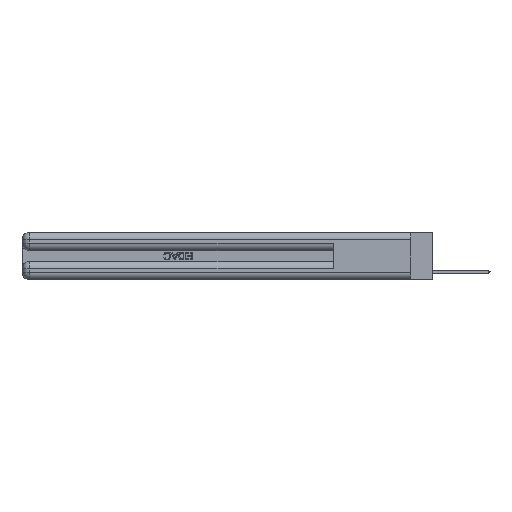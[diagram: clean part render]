
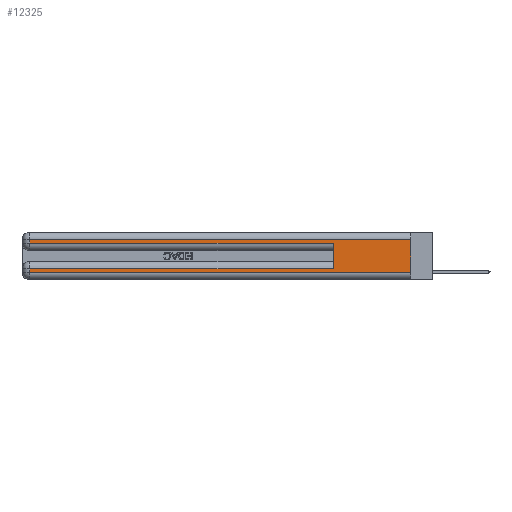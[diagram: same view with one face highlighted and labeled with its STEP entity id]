
A CAD part, left-side view. The second image highlights one B-rep face of the part: STEP entity #12325.
In plain terms, the highlighted planar face has unit normal (-1, 0, 0).
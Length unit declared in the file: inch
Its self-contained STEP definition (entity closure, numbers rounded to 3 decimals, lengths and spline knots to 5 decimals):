
#663 = VERTEX_POINT ( 'NONE', #5618 ) ;
#2014 = VERTEX_POINT ( 'NONE', #27838 ) ;
#2231 = ORIENTED_EDGE ( 'NONE', *, *, #29048, .F. ) ;
#2716 = EDGE_CURVE ( 'NONE', #2014, #30190, #10876, .T. ) ;
#3469 = LINE ( 'NONE', #19719, #8461 ) ;
#3777 = LINE ( 'NONE', #14670, #31603 ) ;
#3831 = DIRECTION ( 'NONE',  ( 0., -1., 0. ) ) ;
#4445 = DIRECTION ( 'NONE',  ( 0., 1., 0. ) ) ;
#5618 = CARTESIAN_POINT ( 'NONE',  ( 0., 0., 0.31 ) ) ;
#5751 = EDGE_CURVE ( 'NONE', #25870, #30190, #3469, .T. ) ;
#5931 = CARTESIAN_POINT ( 'NONE',  ( 0., 0.6, 0.285 ) ) ;
#7234 = EDGE_CURVE ( 'NONE', #28374, #25787, #17374, .T. ) ;
#7680 = VERTEX_POINT ( 'NONE', #26955 ) ;
#7707 = DIRECTION ( 'NONE',  ( 0., 0., -1. ) ) ;
#8461 = VECTOR ( 'NONE', #13833, 39.37008 ) ;
#10499 = EDGE_CURVE ( 'NONE', #2014, #21891, #23003, .T. ) ;
#10876 = LINE ( 'NONE', #21733, #24296 ) ;
#11355 = LINE ( 'NONE', #24713, #13316 ) ;
#11546 = VECTOR ( 'NONE', #28874, 39.37008 ) ;
#11571 = CARTESIAN_POINT ( 'NONE',  ( 0., 2.94, 0.37 ) ) ;
#12023 = ORIENTED_EDGE ( 'NONE', *, *, #2716, .F. ) ;
#12147 = CARTESIAN_POINT ( 'NONE',  ( 0., 2.94, 0.085 ) ) ;
#12325 = ADVANCED_FACE ( 'NONE', ( #22760 ), #25429, .F. ) ;
#12697 = ORIENTED_EDGE ( 'NONE', *, *, #5751, .T. ) ;
#13210 = EDGE_CURVE ( 'NONE', #21891, #28374, #19596, .T. ) ;
#13316 = VECTOR ( 'NONE', #24550, 39.37008 ) ;
#13833 = DIRECTION ( 'NONE',  ( 0., -1., 0. ) ) ;
#14332 = VECTOR ( 'NONE', #4445, 39.37008 ) ;
#14358 = DIRECTION ( 'NONE',  ( 1., 0., 0. ) ) ;
#14670 = CARTESIAN_POINT ( 'NONE',  ( 0., 0., 0.37 ) ) ;
#15573 = DIRECTION ( 'NONE',  ( 0., 0., -1. ) ) ;
#16779 = ORIENTED_EDGE ( 'NONE', *, *, #7234, .T. ) ;
#17032 = DIRECTION ( 'NONE',  ( 0., 0., -1. ) ) ;
#17374 = LINE ( 'NONE', #28254, #25039 ) ;
#19539 = CARTESIAN_POINT ( 'NONE',  ( 0., 2.94, 0.06 ) ) ;
#19596 = LINE ( 'NONE', #11571, #26425 ) ;
#19719 = CARTESIAN_POINT ( 'NONE',  ( 0., 0., 0.285 ) ) ;
#21733 = CARTESIAN_POINT ( 'NONE',  ( 0., 0.6, 0.145 ) ) ;
#21891 = VERTEX_POINT ( 'NONE', #12147 ) ;
#22176 = ORIENTED_EDGE ( 'NONE', *, *, #10499, .T. ) ;
#22388 = CARTESIAN_POINT ( 'NONE',  ( 0., 0., 0.06 ) ) ;
#22760 = FACE_OUTER_BOUND ( 'NONE', #23333, .T. ) ;
#23003 = LINE ( 'NONE', #27961, #14332 ) ;
#23333 = EDGE_LOOP ( 'NONE', ( #2231, #30516, #28028, #12697, #12023, #22176, #31594, #16779 ) ) ;
#24296 = VECTOR ( 'NONE', #32592, 39.37008 ) ;
#24550 = DIRECTION ( 'NONE',  ( 0., 0., -1. ) ) ;
#24652 = EDGE_CURVE ( 'NONE', #663, #7680, #34047, .T. ) ;
#24713 = CARTESIAN_POINT ( 'NONE',  ( 0., 2.94, 0.37 ) ) ;
#25039 = VECTOR ( 'NONE', #3831, 39.37008 ) ;
#25429 = PLANE ( 'NONE',  #26924 ) ;
#25731 = CARTESIAN_POINT ( 'NONE',  ( 0., 2.94, 0.285 ) ) ;
#25787 = VERTEX_POINT ( 'NONE', #22388 ) ;
#25870 = VERTEX_POINT ( 'NONE', #25731 ) ;
#26425 = VECTOR ( 'NONE', #7707, 39.37008 ) ;
#26924 = AXIS2_PLACEMENT_3D ( 'NONE', #28066, #14358, #17032 ) ;
#26955 = CARTESIAN_POINT ( 'NONE',  ( 0., 2.94, 0.31 ) ) ;
#27838 = CARTESIAN_POINT ( 'NONE',  ( 0., 0.6, 0.085 ) ) ;
#27961 = CARTESIAN_POINT ( 'NONE',  ( 0., 0., 0.085 ) ) ;
#28028 = ORIENTED_EDGE ( 'NONE', *, *, #32652, .T. ) ;
#28066 = CARTESIAN_POINT ( 'NONE',  ( 0., 0., 0.37 ) ) ;
#28254 = CARTESIAN_POINT ( 'NONE',  ( 0., 0., 0.06 ) ) ;
#28374 = VERTEX_POINT ( 'NONE', #19539 ) ;
#28502 = CARTESIAN_POINT ( 'NONE',  ( 0., 0., 0.31 ) ) ;
#28874 = DIRECTION ( 'NONE',  ( 0., 1., 0. ) ) ;
#29048 = EDGE_CURVE ( 'NONE', #663, #25787, #3777, .T. ) ;
#30190 = VERTEX_POINT ( 'NONE', #5931 ) ;
#30516 = ORIENTED_EDGE ( 'NONE', *, *, #24652, .T. ) ;
#31594 = ORIENTED_EDGE ( 'NONE', *, *, #13210, .T. ) ;
#31603 = VECTOR ( 'NONE', #15573, 39.37008 ) ;
#32592 = DIRECTION ( 'NONE',  ( 0., 0., 1. ) ) ;
#32652 = EDGE_CURVE ( 'NONE', #7680, #25870, #11355, .T. ) ;
#34047 = LINE ( 'NONE', #28502, #11546 ) ;
